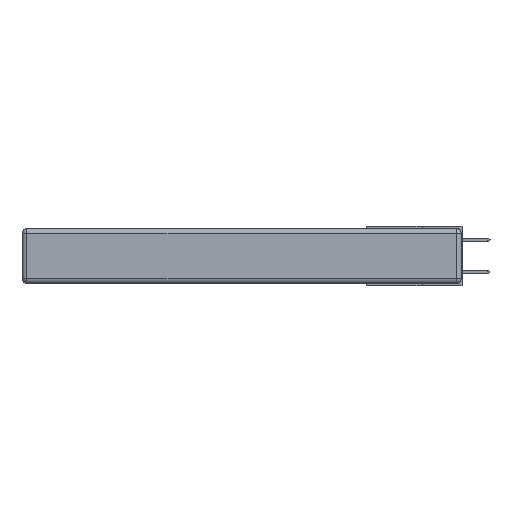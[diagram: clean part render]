
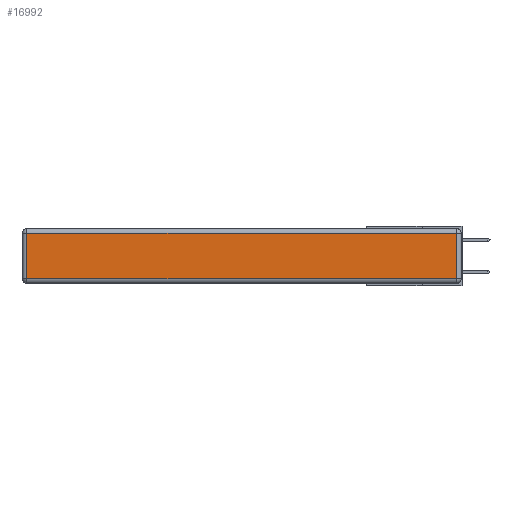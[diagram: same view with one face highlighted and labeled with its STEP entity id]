
A CAD part, left-side view. The second image highlights one B-rep face of the part: STEP entity #16992.
In plain terms, the highlighted planar face has unit normal (-1, 0, 0).
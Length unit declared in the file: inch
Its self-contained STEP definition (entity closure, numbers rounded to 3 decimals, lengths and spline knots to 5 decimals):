
#610 = VECTOR ( 'NONE', #22171, 39.37008 ) ;
#1820 = CARTESIAN_POINT ( 'NONE',  ( 0., 0., -0.313 ) ) ;
#1927 = EDGE_LOOP ( 'NONE', ( #16645, #12100, #16008, #3759 ) ) ;
#2093 = VECTOR ( 'NONE', #4742, 39.37008 ) ;
#3379 = FACE_OUTER_BOUND ( 'NONE', #1927, .T. ) ;
#3759 = ORIENTED_EDGE ( 'NONE', *, *, #18216, .T. ) ;
#4034 = LINE ( 'NONE', #14845, #2093 ) ;
#4101 = PLANE ( 'NONE',  #5113 ) ;
#4742 = DIRECTION ( 'NONE',  ( 0., 0., -1. ) ) ;
#5113 = AXIS2_PLACEMENT_3D ( 'NONE', #16603, #24514, #10113 ) ;
#5843 = VERTEX_POINT ( 'NONE', #11076 ) ;
#6409 = LINE ( 'NONE', #1820, #610 ) ;
#7994 = DIRECTION ( 'NONE',  ( 0., 0., 1. ) ) ;
#8984 = CARTESIAN_POINT ( 'NONE',  ( 0., 2.72, -0.313 ) ) ;
#9204 = EDGE_CURVE ( 'NONE', #9217, #20576, #6409, .T. ) ;
#9217 = VERTEX_POINT ( 'NONE', #8984 ) ;
#10113 = DIRECTION ( 'NONE',  ( 0., 0., 1. ) ) ;
#10549 = CARTESIAN_POINT ( 'NONE',  ( 0., 0.03, -0.313 ) ) ;
#10634 = DIRECTION ( 'NONE',  ( 0., 1., 0. ) ) ;
#11076 = CARTESIAN_POINT ( 'NONE',  ( 0., 2.72, -0.03 ) ) ;
#12100 = ORIENTED_EDGE ( 'NONE', *, *, #13154, .T. ) ;
#12486 = LINE ( 'NONE', #22528, #19143 ) ;
#13054 = VERTEX_POINT ( 'NONE', #18684 ) ;
#13154 = EDGE_CURVE ( 'NONE', #20576, #13054, #12486, .T. ) ;
#14480 = CARTESIAN_POINT ( 'NONE',  ( 0., 2.75, -0.03 ) ) ;
#14845 = CARTESIAN_POINT ( 'NONE',  ( 0., 2.72, -0.343 ) ) ;
#16008 = ORIENTED_EDGE ( 'NONE', *, *, #21984, .T. ) ;
#16603 = CARTESIAN_POINT ( 'NONE',  ( 0., 0., -0.343 ) ) ;
#16645 = ORIENTED_EDGE ( 'NONE', *, *, #9204, .T. ) ;
#16992 = ADVANCED_FACE ( 'NONE', ( #3379 ), #4101, .T. ) ;
#17213 = LINE ( 'NONE', #14480, #25169 ) ;
#18216 = EDGE_CURVE ( 'NONE', #5843, #9217, #4034, .T. ) ;
#18684 = CARTESIAN_POINT ( 'NONE',  ( 0., 0.03, -0.03 ) ) ;
#19143 = VECTOR ( 'NONE', #7994, 39.37008 ) ;
#20576 = VERTEX_POINT ( 'NONE', #10549 ) ;
#21984 = EDGE_CURVE ( 'NONE', #13054, #5843, #17213, .T. ) ;
#22171 = DIRECTION ( 'NONE',  ( 0., -1., 0. ) ) ;
#22528 = CARTESIAN_POINT ( 'NONE',  ( 0., 0.03, -0.343 ) ) ;
#24514 = DIRECTION ( 'NONE',  ( -1., 0., 0. ) ) ;
#25169 = VECTOR ( 'NONE', #10634, 39.37008 ) ;
